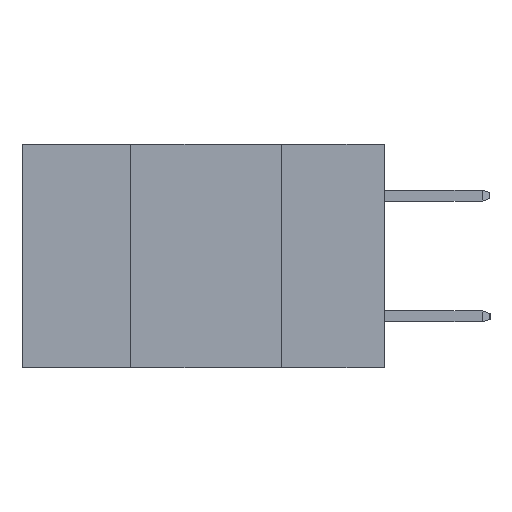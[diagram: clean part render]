
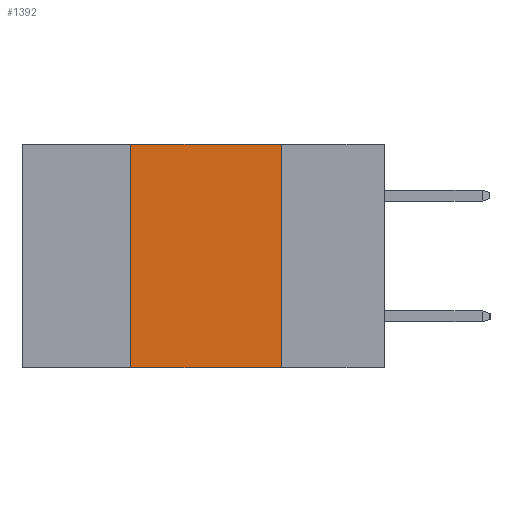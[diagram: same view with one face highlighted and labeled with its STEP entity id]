
A CAD part, left-side view. The second image highlights one B-rep face of the part: STEP entity #1392.
In plain terms, the highlighted planar face has unit normal (-1, 0, 0).
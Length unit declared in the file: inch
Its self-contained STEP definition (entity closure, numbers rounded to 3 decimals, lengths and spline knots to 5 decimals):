
#498 = CARTESIAN_POINT ( 'NONE',  ( 0., 0.6, -0.37 ) ) ;
#635 = DIRECTION ( 'NONE',  ( 0., -1., 0. ) ) ;
#654 = VERTEX_POINT ( 'NONE', #10178 ) ;
#655 = VECTOR ( 'NONE', #635, 39.37008 ) ;
#1392 = ADVANCED_FACE ( 'NONE', ( #2969 ), #7290, .F. ) ;
#1982 = DIRECTION ( 'NONE',  ( 0., -1., 0. ) ) ;
#2043 = CARTESIAN_POINT ( 'NONE',  ( 0., 0.6, 0. ) ) ;
#2340 = LINE ( 'NONE', #9050, #8173 ) ;
#2793 = CARTESIAN_POINT ( 'NONE',  ( 0., 0.17, 0. ) ) ;
#2969 = FACE_OUTER_BOUND ( 'NONE', #3039, .T. ) ;
#3039 = EDGE_LOOP ( 'NONE', ( #4711, #10329, #8228, #8881 ) ) ;
#3163 = VERTEX_POINT ( 'NONE', #10678 ) ;
#3670 = DIRECTION ( 'NONE',  ( 0., 0., -1. ) ) ;
#4422 = VERTEX_POINT ( 'NONE', #2793 ) ;
#4711 = ORIENTED_EDGE ( 'NONE', *, *, #13544, .F. ) ;
#5172 = VECTOR ( 'NONE', #1982, 39.37008 ) ;
#5371 = DIRECTION ( 'NONE',  ( 1., 0., 0. ) ) ;
#5933 = AXIS2_PLACEMENT_3D ( 'NONE', #6839, #5371, #3670 ) ;
#6124 = LINE ( 'NONE', #498, #655 ) ;
#6449 = CARTESIAN_POINT ( 'NONE',  ( 0., 0.42, 0. ) ) ;
#6839 = CARTESIAN_POINT ( 'NONE',  ( 0., 0.6, 0. ) ) ;
#7290 = PLANE ( 'NONE',  #5933 ) ;
#7943 = EDGE_CURVE ( 'NONE', #3163, #654, #6124, .T. ) ;
#8038 = LINE ( 'NONE', #2043, #5172 ) ;
#8173 = VECTOR ( 'NONE', #8916, 39.37008 ) ;
#8228 = ORIENTED_EDGE ( 'NONE', *, *, #10014, .F. ) ;
#8392 = LINE ( 'NONE', #11168, #13642 ) ;
#8881 = ORIENTED_EDGE ( 'NONE', *, *, #7943, .T. ) ;
#8916 = DIRECTION ( 'NONE',  ( 0., 0., -1. ) ) ;
#9050 = CARTESIAN_POINT ( 'NONE',  ( 0., 0.17, -0.37 ) ) ;
#10014 = EDGE_CURVE ( 'NONE', #3163, #10701, #8392, .T. ) ;
#10178 = CARTESIAN_POINT ( 'NONE',  ( 0., 0.17, -0.37 ) ) ;
#10329 = ORIENTED_EDGE ( 'NONE', *, *, #12870, .F. ) ;
#10678 = CARTESIAN_POINT ( 'NONE',  ( 0., 0.42, -0.37 ) ) ;
#10701 = VERTEX_POINT ( 'NONE', #6449 ) ;
#11117 = DIRECTION ( 'NONE',  ( 0., 0., 1. ) ) ;
#11168 = CARTESIAN_POINT ( 'NONE',  ( 0., 0.42, -0.37 ) ) ;
#12870 = EDGE_CURVE ( 'NONE', #10701, #4422, #8038, .T. ) ;
#13544 = EDGE_CURVE ( 'NONE', #4422, #654, #2340, .T. ) ;
#13642 = VECTOR ( 'NONE', #11117, 39.37008 ) ;
